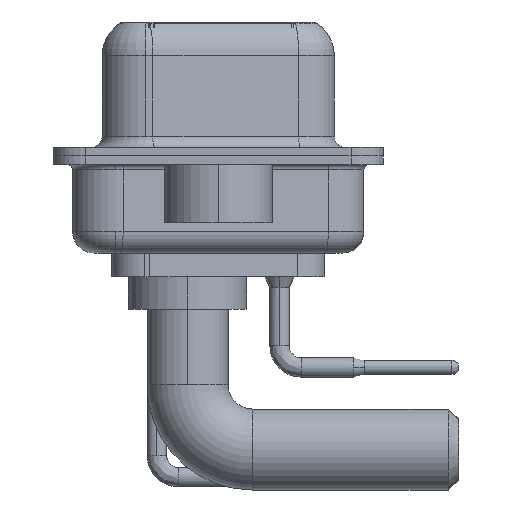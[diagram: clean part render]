
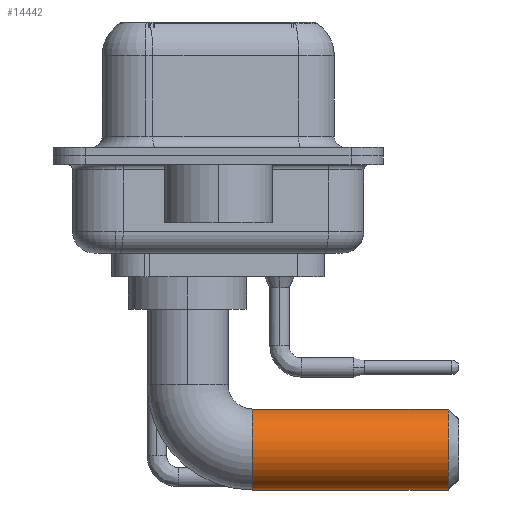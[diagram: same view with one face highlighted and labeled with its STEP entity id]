
A CAD part, left-side view. The second image highlights one B-rep face of the part: STEP entity #14442.
In plain terms, the highlighted cylindrical face has radius 1.875 mm (diameter 3.75 mm), a partial arc.
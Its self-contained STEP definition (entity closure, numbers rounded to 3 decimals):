
#315 = CARTESIAN_POINT ( 'NONE',  ( 0., -3., -4.625 ) ) ;
#1182 = ORIENTED_EDGE ( 'NONE', *, *, #27425, .T. ) ;
#1406 = EDGE_CURVE ( 'NONE', #4738, #7096, #32117, .T. ) ;
#1408 = DIRECTION ( 'NONE',  ( 0., 1., 0. ) ) ;
#1594 = EDGE_CURVE ( 'NONE', #22485, #8881, #24745, .T. ) ;
#3377 = ORIENTED_EDGE ( 'NONE', *, *, #25521, .T. ) ;
#4359 = CYLINDRICAL_SURFACE ( 'NONE', #27705, 1.875 ) ;
#4738 = VERTEX_POINT ( 'NONE', #26677 ) ;
#6773 = CARTESIAN_POINT ( 'NONE',  ( 0., -3., -6.5 ) ) ;
#7096 = VERTEX_POINT ( 'NONE', #14288 ) ;
#8442 = AXIS2_PLACEMENT_3D ( 'NONE', #24984, #1408, #11893 ) ;
#8881 = VERTEX_POINT ( 'NONE', #26959 ) ;
#10302 = DIRECTION ( 'NONE',  ( -1., 0., 0. ) ) ;
#11893 = DIRECTION ( 'NONE',  ( 0., 0., -1. ) ) ;
#11937 = DIRECTION ( 'NONE',  ( 0., 0., -1. ) ) ;
#12877 = CARTESIAN_POINT ( 'NONE',  ( 0., -3., -6.5 ) ) ;
#13519 = AXIS2_PLACEMENT_3D ( 'NONE', #12877, #15878, #10302 ) ;
#14228 = DIRECTION ( 'NONE',  ( 0., -1., 0. ) ) ;
#14288 = CARTESIAN_POINT ( 'NONE',  ( 0., -12.07, -4.625 ) ) ;
#14442 = ADVANCED_FACE ( 'NONE', ( #20211 ), #4359, .T. ) ;
#15878 = DIRECTION ( 'NONE',  ( 0., -1., 0. ) ) ;
#17168 = CARTESIAN_POINT ( 'NONE',  ( 0., -3., -8.375 ) ) ;
#19584 = VECTOR ( 'NONE', #14228, 1000. ) ;
#19848 = ORIENTED_EDGE ( 'NONE', *, *, #1406, .F. ) ;
#20211 = FACE_OUTER_BOUND ( 'NONE', #31531, .T. ) ;
#21019 = ORIENTED_EDGE ( 'NONE', *, *, #1594, .T. ) ;
#22485 = VERTEX_POINT ( 'NONE', #30824 ) ;
#24391 = CIRCLE ( 'NONE', #8442, 1.875 ) ;
#24745 = LINE ( 'NONE', #17168, #19584 ) ;
#24984 = CARTESIAN_POINT ( 'NONE',  ( 0., -12.07, -6.5 ) ) ;
#25521 = EDGE_CURVE ( 'NONE', #8881, #7096, #24391, .T. ) ;
#26139 = DIRECTION ( 'NONE',  ( 0., -1., 0. ) ) ;
#26677 = CARTESIAN_POINT ( 'NONE',  ( 0., -3., -4.625 ) ) ;
#26959 = CARTESIAN_POINT ( 'NONE',  ( 0., -12.07, -8.375 ) ) ;
#27425 = EDGE_CURVE ( 'NONE', #4738, #22485, #28903, .T. ) ;
#27705 = AXIS2_PLACEMENT_3D ( 'NONE', #6773, #27757, #11937 ) ;
#27757 = DIRECTION ( 'NONE',  ( 0., -1., 0. ) ) ;
#28903 = CIRCLE ( 'NONE', #13519, 1.875 ) ;
#30824 = CARTESIAN_POINT ( 'NONE',  ( 0., -3., -8.375 ) ) ;
#31531 = EDGE_LOOP ( 'NONE', ( #19848, #1182, #21019, #3377 ) ) ;
#32117 = LINE ( 'NONE', #315, #33867 ) ;
#33867 = VECTOR ( 'NONE', #26139, 1000. ) ;
